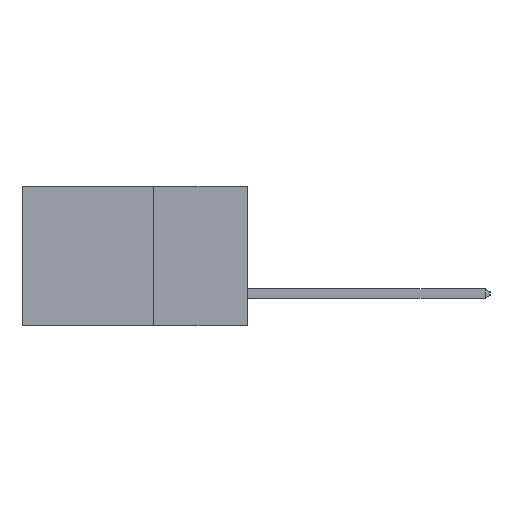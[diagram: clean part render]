
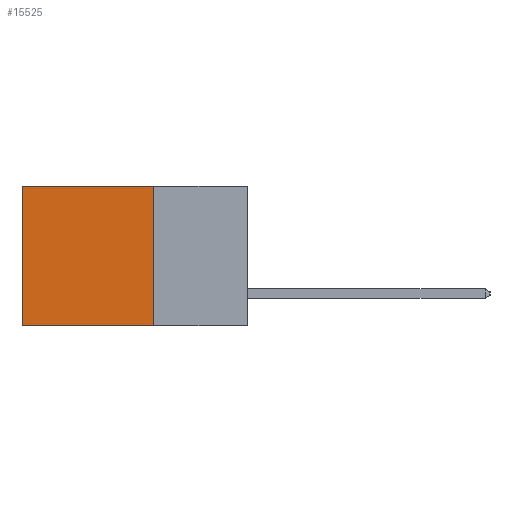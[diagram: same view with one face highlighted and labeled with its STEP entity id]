
A CAD part, left-side view. The second image highlights one B-rep face of the part: STEP entity #15525.
In plain terms, the highlighted planar face has unit normal (-1, 0, 0).
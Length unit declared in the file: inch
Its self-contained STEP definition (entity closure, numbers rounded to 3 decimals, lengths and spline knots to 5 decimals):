
#2604 = CARTESIAN_POINT ( 'NONE',  ( 0.298, 0.25, 0. ) ) ;
#3669 = CARTESIAN_POINT ( 'NONE',  ( 0.298, 0.6, -0.37 ) ) ;
#4665 = LINE ( 'NONE', #19849, #16904 ) ;
#4847 = ORIENTED_EDGE ( 'NONE', *, *, #13644, .F. ) ;
#5111 = EDGE_CURVE ( 'NONE', #23157, #12579, #11928, .T. ) ;
#5608 = CARTESIAN_POINT ( 'NONE',  ( 0.298, 0.6, 0. ) ) ;
#6205 = DIRECTION ( 'NONE',  ( 0., 0., -1. ) ) ;
#7134 = PLANE ( 'NONE',  #7726 ) ;
#7284 = CARTESIAN_POINT ( 'NONE',  ( 0.298, 0.25, 0. ) ) ;
#7726 = AXIS2_PLACEMENT_3D ( 'NONE', #16303, #27386, #14129 ) ;
#7729 = EDGE_CURVE ( 'NONE', #29231, #23497, #10633, .T. ) ;
#9158 = ORIENTED_EDGE ( 'NONE', *, *, #7729, .T. ) ;
#10282 = DIRECTION ( 'NONE',  ( 0., 1., 0. ) ) ;
#10633 = LINE ( 'NONE', #28024, #27731 ) ;
#11163 = EDGE_LOOP ( 'NONE', ( #18201, #18207, #4847, #9158 ) ) ;
#11421 = CARTESIAN_POINT ( 'NONE',  ( 0.298, 0.25, -0.37 ) ) ;
#11928 = LINE ( 'NONE', #22222, #28931 ) ;
#12579 = VERTEX_POINT ( 'NONE', #3669 ) ;
#13644 = EDGE_CURVE ( 'NONE', #29231, #23157, #14903, .T. ) ;
#14129 = DIRECTION ( 'NONE',  ( 0., 0., -1. ) ) ;
#14903 = LINE ( 'NONE', #2604, #25303 ) ;
#15525 = ADVANCED_FACE ( 'NONE', ( #27294 ), #7134, .F. ) ;
#16303 = CARTESIAN_POINT ( 'NONE',  ( 0.298, 0.25, 0. ) ) ;
#16904 = VECTOR ( 'NONE', #6205, 39.37008 ) ;
#18201 = ORIENTED_EDGE ( 'NONE', *, *, #23627, .T. ) ;
#18207 = ORIENTED_EDGE ( 'NONE', *, *, #5111, .F. ) ;
#19849 = CARTESIAN_POINT ( 'NONE',  ( 0.298, 0.6, 0. ) ) ;
#20874 = DIRECTION ( 'NONE',  ( 0., 0., -1. ) ) ;
#22222 = CARTESIAN_POINT ( 'NONE',  ( 0.298, 0.25, -0.37 ) ) ;
#23157 = VERTEX_POINT ( 'NONE', #11421 ) ;
#23497 = VERTEX_POINT ( 'NONE', #5608 ) ;
#23627 = EDGE_CURVE ( 'NONE', #23497, #12579, #4665, .T. ) ;
#25303 = VECTOR ( 'NONE', #20874, 39.37008 ) ;
#26682 = DIRECTION ( 'NONE',  ( 0., 1., 0. ) ) ;
#27294 = FACE_OUTER_BOUND ( 'NONE', #11163, .T. ) ;
#27386 = DIRECTION ( 'NONE',  ( 1., 0., 0. ) ) ;
#27731 = VECTOR ( 'NONE', #10282, 39.37008 ) ;
#28024 = CARTESIAN_POINT ( 'NONE',  ( 0.298, 0.25, 0. ) ) ;
#28931 = VECTOR ( 'NONE', #26682, 39.37008 ) ;
#29231 = VERTEX_POINT ( 'NONE', #7284 ) ;
